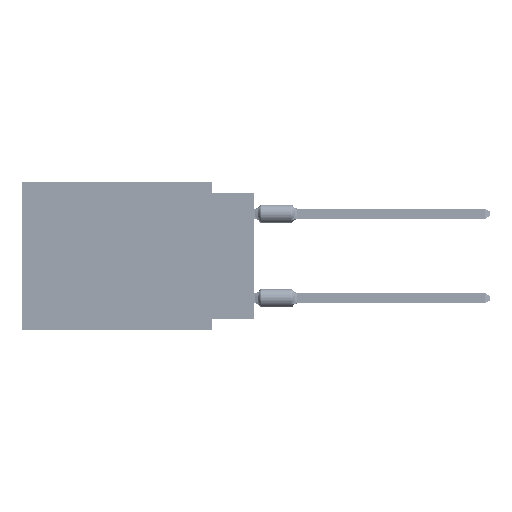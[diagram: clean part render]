
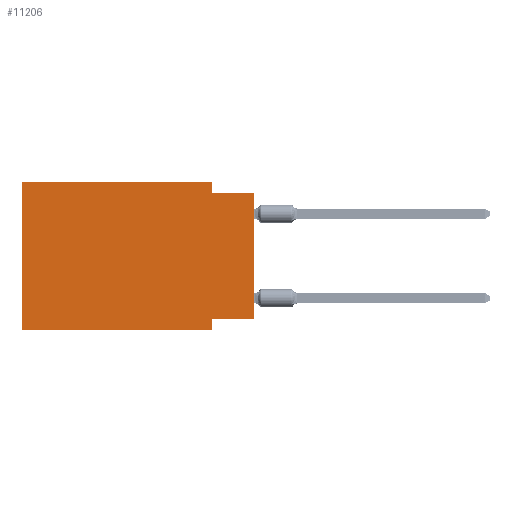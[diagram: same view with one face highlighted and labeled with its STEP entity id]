
A CAD part, left-side view. The second image highlights one B-rep face of the part: STEP entity #11206.
In plain terms, the highlighted planar face has unit normal (-1, 0, 0).
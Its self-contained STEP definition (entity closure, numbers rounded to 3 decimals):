
#269 = CARTESIAN_POINT ( 'NONE',  ( 0., 0., -0.635 ) ) ;
#418 = LINE ( 'NONE', #22401, #9002 ) ;
#1874 = VECTOR ( 'NONE', #100048, 1000. ) ;
#3495 = DIRECTION ( 'NONE',  ( 0., 0., -1. ) ) ;
#3907 = VECTOR ( 'NONE', #60355, 1000. ) ;
#9002 = VECTOR ( 'NONE', #55670, 1000. ) ;
#10425 = DIRECTION ( 'NONE',  ( 0., 0., 1. ) ) ;
#11143 = LINE ( 'NONE', #18802, #92567 ) ;
#11206 = ADVANCED_FACE ( 'NONE', ( #29499 ), #62253, .F. ) ;
#11467 = CARTESIAN_POINT ( 'NONE',  ( 0., 13.97, 0. ) ) ;
#13671 = VERTEX_POINT ( 'NONE', #11467 ) ;
#18802 = CARTESIAN_POINT ( 'NONE',  ( 0., 2.54, 0. ) ) ;
#19167 = CARTESIAN_POINT ( 'NONE',  ( 0., 0., -8.255 ) ) ;
#20254 = CARTESIAN_POINT ( 'NONE',  ( 0., 13.97, 0. ) ) ;
#21640 = ORIENTED_EDGE ( 'NONE', *, *, #26933, .F. ) ;
#22401 = CARTESIAN_POINT ( 'NONE',  ( 0., 2.54, -8.89 ) ) ;
#24911 = VECTOR ( 'NONE', #33032, 1000. ) ;
#26933 = EDGE_CURVE ( 'NONE', #78708, #13671, #67968, .T. ) ;
#29499 = FACE_OUTER_BOUND ( 'NONE', #66045, .T. ) ;
#31421 = CARTESIAN_POINT ( 'NONE',  ( 0., 13.97, 0. ) ) ;
#33032 = DIRECTION ( 'NONE',  ( 0., -1., 0. ) ) ;
#35266 = CARTESIAN_POINT ( 'NONE',  ( 0., 0., -8.255 ) ) ;
#36532 = AXIS2_PLACEMENT_3D ( 'NONE', #20254, #95505, #77527 ) ;
#40215 = CARTESIAN_POINT ( 'NONE',  ( 0., 2.54, -8.255 ) ) ;
#42341 = DIRECTION ( 'NONE',  ( 0., 0., 1. ) ) ;
#42876 = CARTESIAN_POINT ( 'NONE',  ( 0., 13.97, 0. ) ) ;
#43433 = LINE ( 'NONE', #35266, #3907 ) ;
#44937 = VECTOR ( 'NONE', #42341, 1000. ) ;
#45527 = VERTEX_POINT ( 'NONE', #19167 ) ;
#46196 = VERTEX_POINT ( 'NONE', #40215 ) ;
#46322 = EDGE_CURVE ( 'NONE', #45527, #46196, #43433, .T. ) ;
#46850 = ORIENTED_EDGE ( 'NONE', *, *, #104918, .F. ) ;
#51871 = CARTESIAN_POINT ( 'NONE',  ( 0., 0., 0. ) ) ;
#54485 = ORIENTED_EDGE ( 'NONE', *, *, #46322, .F. ) ;
#55598 = VERTEX_POINT ( 'NONE', #62493 ) ;
#55670 = DIRECTION ( 'NONE',  ( 0., 0., -1. ) ) ;
#57887 = CARTESIAN_POINT ( 'NONE',  ( 0., 0., -0.635 ) ) ;
#60059 = LINE ( 'NONE', #51871, #74146 ) ;
#60355 = DIRECTION ( 'NONE',  ( 0., 1., 0. ) ) ;
#62253 = PLANE ( 'NONE',  #36532 ) ;
#62493 = CARTESIAN_POINT ( 'NONE',  ( 0., 2.54, -0.635 ) ) ;
#62760 = EDGE_CURVE ( 'NONE', #78708, #95485, #65422, .T. ) ;
#63508 = ORIENTED_EDGE ( 'NONE', *, *, #101918, .F. ) ;
#65422 = LINE ( 'NONE', #82861, #95500 ) ;
#66045 = EDGE_LOOP ( 'NONE', ( #69809, #63508, #46850, #68032, #21640, #95135, #67945, #54485 ) ) ;
#67945 = ORIENTED_EDGE ( 'NONE', *, *, #83372, .F. ) ;
#67968 = LINE ( 'NONE', #42876, #44937 ) ;
#68032 = ORIENTED_EDGE ( 'NONE', *, *, #106457, .F. ) ;
#68519 = CARTESIAN_POINT ( 'NONE',  ( 0., 2.54, -8.89 ) ) ;
#69809 = ORIENTED_EDGE ( 'NONE', *, *, #91287, .T. ) ;
#73368 = LINE ( 'NONE', #269, #1874 ) ;
#74146 = VECTOR ( 'NONE', #10425, 1000. ) ;
#75232 = DIRECTION ( 'NONE',  ( 0., -1., 0. ) ) ;
#76446 = CARTESIAN_POINT ( 'NONE',  ( 0., 13.97, -8.89 ) ) ;
#77527 = DIRECTION ( 'NONE',  ( 0., 0., -1. ) ) ;
#78708 = VERTEX_POINT ( 'NONE', #76446 ) ;
#82861 = CARTESIAN_POINT ( 'NONE',  ( 0., 13.97, -8.89 ) ) ;
#83248 = CARTESIAN_POINT ( 'NONE',  ( 0., 2.54, 0. ) ) ;
#83372 = EDGE_CURVE ( 'NONE', #46196, #95485, #418, .T. ) ;
#91287 = EDGE_CURVE ( 'NONE', #45527, #93183, #60059, .T. ) ;
#92567 = VECTOR ( 'NONE', #3495, 1000. ) ;
#93183 = VERTEX_POINT ( 'NONE', #57887 ) ;
#95135 = ORIENTED_EDGE ( 'NONE', *, *, #62760, .T. ) ;
#95485 = VERTEX_POINT ( 'NONE', #68519 ) ;
#95500 = VECTOR ( 'NONE', #75232, 1000. ) ;
#95505 = DIRECTION ( 'NONE',  ( 1., 0., 0. ) ) ;
#99318 = VERTEX_POINT ( 'NONE', #83248 ) ;
#100048 = DIRECTION ( 'NONE',  ( 0., -1., 0. ) ) ;
#101918 = EDGE_CURVE ( 'NONE', #55598, #93183, #73368, .T. ) ;
#104918 = EDGE_CURVE ( 'NONE', #99318, #55598, #11143, .T. ) ;
#106110 = LINE ( 'NONE', #31421, #24911 ) ;
#106457 = EDGE_CURVE ( 'NONE', #13671, #99318, #106110, .T. ) ;
